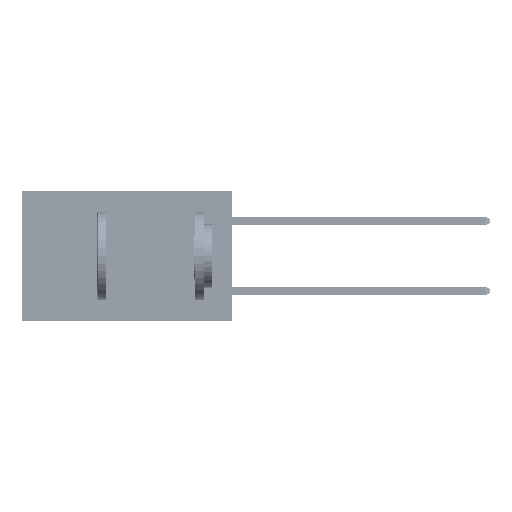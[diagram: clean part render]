
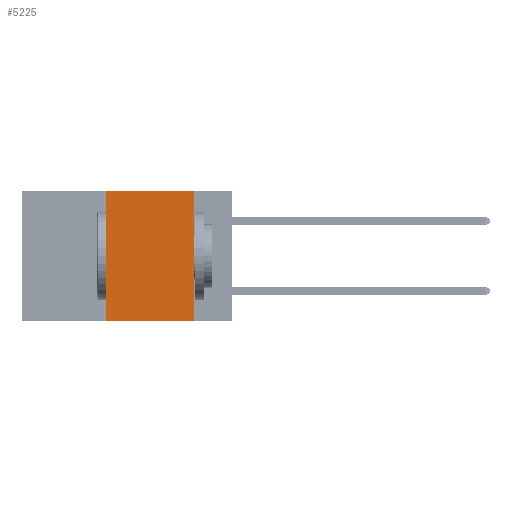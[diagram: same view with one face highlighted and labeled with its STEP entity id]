
A CAD part, left-side view. The second image highlights one B-rep face of the part: STEP entity #5225.
In plain terms, the highlighted planar face has unit normal (-1, 0, 0).
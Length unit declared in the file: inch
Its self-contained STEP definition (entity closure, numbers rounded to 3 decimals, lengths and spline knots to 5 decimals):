
#133 = CARTESIAN_POINT ( 'NONE',  ( 0., 0.6, -0.37 ) ) ;
#1327 = CARTESIAN_POINT ( 'NONE',  ( 0., 0.11, 0. ) ) ;
#2400 = CARTESIAN_POINT ( 'NONE',  ( 0., 0.36, -0.37 ) ) ;
#2550 = DIRECTION ( 'NONE',  ( 0., 0., -1. ) ) ;
#4071 = VECTOR ( 'NONE', #37022, 39.37008 ) ;
#4557 = EDGE_CURVE ( 'NONE', #11166, #28310, #40719, .T. ) ;
#4653 = DIRECTION ( 'NONE',  ( 0., -1., 0. ) ) ;
#4722 = VERTEX_POINT ( 'NONE', #10564 ) ;
#5225 = ADVANCED_FACE ( 'NONE', ( #47423 ), #12830, .F. ) ;
#6444 = VECTOR ( 'NONE', #48231, 39.37008 ) ;
#8732 = VECTOR ( 'NONE', #2550, 39.37008 ) ;
#9117 = VERTEX_POINT ( 'NONE', #2400 ) ;
#10564 = CARTESIAN_POINT ( 'NONE',  ( 0., 0.36, 0. ) ) ;
#11166 = VERTEX_POINT ( 'NONE', #49368 ) ;
#11259 = CARTESIAN_POINT ( 'NONE',  ( 0., 0.11, -0.37 ) ) ;
#12516 = CARTESIAN_POINT ( 'NONE',  ( 0., 0.36, 0. ) ) ;
#12830 = PLANE ( 'NONE',  #37468 ) ;
#14045 = EDGE_CURVE ( 'NONE', #4722, #11166, #36618, .T. ) ;
#14757 = LINE ( 'NONE', #12516, #4071 ) ;
#14906 = VECTOR ( 'NONE', #4653, 39.37008 ) ;
#17014 = DIRECTION ( 'NONE',  ( 1., 0., 0. ) ) ;
#20309 = CARTESIAN_POINT ( 'NONE',  ( 0., 0.6, 0. ) ) ;
#22219 = ORIENTED_EDGE ( 'NONE', *, *, #4557, .F. ) ;
#23269 = EDGE_LOOP ( 'NONE', ( #22219, #32417, #39227, #23326 ) ) ;
#23326 = ORIENTED_EDGE ( 'NONE', *, *, #47631, .T. ) ;
#24326 = LINE ( 'NONE', #133, #14906 ) ;
#24797 = EDGE_CURVE ( 'NONE', #9117, #4722, #14757, .T. ) ;
#28310 = VERTEX_POINT ( 'NONE', #11259 ) ;
#32417 = ORIENTED_EDGE ( 'NONE', *, *, #14045, .F. ) ;
#32965 = CARTESIAN_POINT ( 'NONE',  ( 0., 0.6, 0. ) ) ;
#33313 = DIRECTION ( 'NONE',  ( 0., 0., -1. ) ) ;
#36618 = LINE ( 'NONE', #20309, #6444 ) ;
#37022 = DIRECTION ( 'NONE',  ( 0., 0., 1. ) ) ;
#37468 = AXIS2_PLACEMENT_3D ( 'NONE', #32965, #17014, #33313 ) ;
#39227 = ORIENTED_EDGE ( 'NONE', *, *, #24797, .F. ) ;
#40719 = LINE ( 'NONE', #1327, #8732 ) ;
#47423 = FACE_OUTER_BOUND ( 'NONE', #23269, .T. ) ;
#47631 = EDGE_CURVE ( 'NONE', #9117, #28310, #24326, .T. ) ;
#48231 = DIRECTION ( 'NONE',  ( 0., -1., 0. ) ) ;
#49368 = CARTESIAN_POINT ( 'NONE',  ( 0., 0.11, 0. ) ) ;
